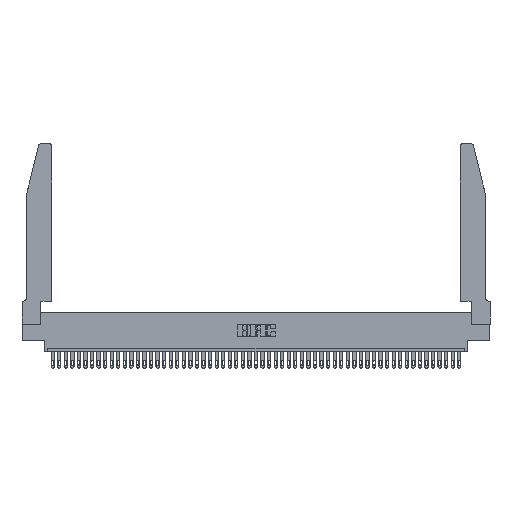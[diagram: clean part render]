
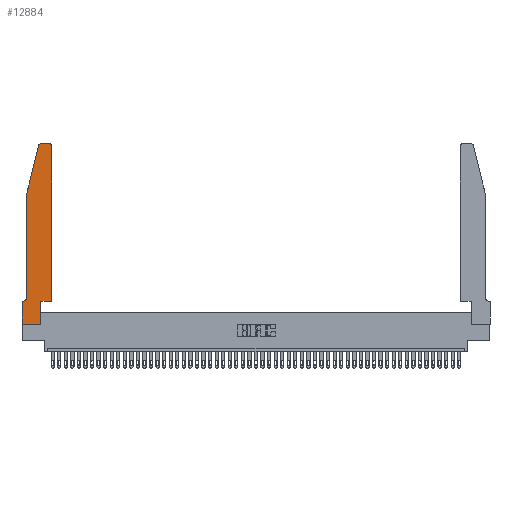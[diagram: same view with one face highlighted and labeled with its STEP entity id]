
A CAD part, top view. The second image highlights one B-rep face of the part: STEP entity #12884.
In plain terms, the highlighted planar face has unit normal (0, 0, 1).
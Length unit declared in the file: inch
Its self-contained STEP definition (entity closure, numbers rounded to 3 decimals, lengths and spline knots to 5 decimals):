
#888 = VERTEX_POINT ( 'NONE', #4504 ) ;
#1213 = DIRECTION ( 'NONE',  ( 0., -1., 0. ) ) ;
#1390 = CIRCLE ( 'NONE', #10165, 0.03 ) ;
#1454 = EDGE_CURVE ( 'NONE', #31015, #30696, #16986, .T. ) ;
#2493 = DIRECTION ( 'NONE',  ( 0., 0., 1. ) ) ;
#2684 = DIRECTION ( 'NONE',  ( 1., 0., 0. ) ) ;
#2699 = ORIENTED_EDGE ( 'NONE', *, *, #43784, .T. ) ;
#3818 = AXIS2_PLACEMENT_3D ( 'NONE', #6189, #2493, #9884 ) ;
#4504 = CARTESIAN_POINT ( 'NONE',  ( 0., 0.35, 0.37 ) ) ;
#4913 = ORIENTED_EDGE ( 'NONE', *, *, #13318, .T. ) ;
#5600 = VECTOR ( 'NONE', #31798, 39.37008 ) ;
#5611 = LINE ( 'NONE', #37325, #37312 ) ;
#5988 = VERTEX_POINT ( 'NONE', #7144 ) ;
#5996 = CARTESIAN_POINT ( 'NONE',  ( 0.0755, 0.42, 0.37 ) ) ;
#6189 = CARTESIAN_POINT ( 'NONE',  ( 0.284, 2.72, 0.37 ) ) ;
#6255 = EDGE_CURVE ( 'NONE', #40191, #6283, #39268, .T. ) ;
#6283 = VERTEX_POINT ( 'NONE', #18095 ) ;
#6309 = DIRECTION ( 'NONE',  ( 1., 0., 0. ) ) ;
#6886 = LINE ( 'NONE', #18804, #15251 ) ;
#7144 = CARTESIAN_POINT ( 'NONE',  ( 0.0055, 0.35, 0.37 ) ) ;
#7612 = CARTESIAN_POINT ( 'NONE',  ( 0.2865, 0., 0.37 ) ) ;
#8094 = EDGE_CURVE ( 'NONE', #49021, #15102, #6886, .T. ) ;
#8491 = CARTESIAN_POINT ( 'NONE',  ( 0.4505, 0.35, 0.37 ) ) ;
#8656 = LINE ( 'NONE', #8491, #48115 ) ;
#8812 = VECTOR ( 'NONE', #42785, 39.37008 ) ;
#9861 = EDGE_CURVE ( 'NONE', #43512, #14122, #1390, .T. ) ;
#9884 = DIRECTION ( 'NONE',  ( 1., 0., 0. ) ) ;
#10165 = AXIS2_PLACEMENT_3D ( 'NONE', #17005, #29199, #6309 ) ;
#10758 = VECTOR ( 'NONE', #1213, 39.37008 ) ;
#11396 = AXIS2_PLACEMENT_3D ( 'NONE', #46126, #45983, #34969 ) ;
#11564 = CARTESIAN_POINT ( 'NONE',  ( 0.0755, 2., 0.37 ) ) ;
#12884 = ADVANCED_FACE ( 'NONE', ( #32865 ), #49000, .T. ) ;
#13318 = EDGE_CURVE ( 'NONE', #888, #31015, #15512, .T. ) ;
#14122 = VERTEX_POINT ( 'NONE', #23144 ) ;
#14564 = CARTESIAN_POINT ( 'NONE',  ( 0.2865, 0.35, 0.37 ) ) ;
#14869 = VECTOR ( 'NONE', #49241, 39.37008 ) ;
#15102 = VERTEX_POINT ( 'NONE', #11564 ) ;
#15251 = VECTOR ( 'NONE', #37318, 39.37008 ) ;
#15512 = LINE ( 'NONE', #32156, #10758 ) ;
#16405 = VECTOR ( 'NONE', #33693, 39.37008 ) ;
#16986 = LINE ( 'NONE', #24149, #5600 ) ;
#17005 = CARTESIAN_POINT ( 'NONE',  ( 0.4205, 2.72, 0.37 ) ) ;
#17025 = EDGE_CURVE ( 'NONE', #6283, #43512, #8656, .T. ) ;
#17609 = DIRECTION ( 'NONE',  ( 0., 0., 1. ) ) ;
#17669 = LINE ( 'NONE', #14564, #16405 ) ;
#18095 = CARTESIAN_POINT ( 'NONE',  ( 0.4505, 0.35, 0.37 ) ) ;
#18153 = CARTESIAN_POINT ( 'NONE',  ( 0.0755, 0.35, 0.37 ) ) ;
#18410 = CARTESIAN_POINT ( 'NONE',  ( 0.2865, 0.35, 0.37 ) ) ;
#18804 = CARTESIAN_POINT ( 'NONE',  ( 0.0755, 2., 0.37 ) ) ;
#19162 = CIRCLE ( 'NONE', #11396, 0.07 ) ;
#19190 = ORIENTED_EDGE ( 'NONE', *, *, #24174, .T. ) ;
#19346 = CARTESIAN_POINT ( 'NONE',  ( 0.25487, 2.72718, 0.37 ) ) ;
#19467 = CARTESIAN_POINT ( 'NONE',  ( 0., 0.35, 0.37 ) ) ;
#20998 = ORIENTED_EDGE ( 'NONE', *, *, #32439, .T. ) ;
#21939 = LINE ( 'NONE', #18153, #40977 ) ;
#21992 = DIRECTION ( 'NONE',  ( -1., 0., 0. ) ) ;
#23144 = CARTESIAN_POINT ( 'NONE',  ( 0.4205, 2.75, 0.37 ) ) ;
#24149 = CARTESIAN_POINT ( 'NONE',  ( 0., 0., 0.37 ) ) ;
#24174 = EDGE_CURVE ( 'NONE', #30195, #49021, #41210, .T. ) ;
#24372 = CARTESIAN_POINT ( 'NONE',  ( 0.4505, 0.35, 0.37 ) ) ;
#26081 = EDGE_CURVE ( 'NONE', #5988, #888, #21939, .T. ) ;
#26747 = ORIENTED_EDGE ( 'NONE', *, *, #8094, .T. ) ;
#26897 = ORIENTED_EDGE ( 'NONE', *, *, #41486, .T. ) ;
#28063 = CARTESIAN_POINT ( 'NONE',  ( 0., 0., 0.37 ) ) ;
#28498 = AXIS2_PLACEMENT_3D ( 'NONE', #19467, #17609, #2684 ) ;
#28583 = DIRECTION ( 'NONE',  ( 0., 1., 0. ) ) ;
#29199 = DIRECTION ( 'NONE',  ( 0., 0., 1. ) ) ;
#29377 = ORIENTED_EDGE ( 'NONE', *, *, #1454, .T. ) ;
#30195 = VERTEX_POINT ( 'NONE', #48517 ) ;
#30696 = VERTEX_POINT ( 'NONE', #7612 ) ;
#31015 = VERTEX_POINT ( 'NONE', #28063 ) ;
#31034 = EDGE_CURVE ( 'NONE', #15102, #44499, #39200, .T. ) ;
#31492 = EDGE_LOOP ( 'NONE', ( #26897, #19190, #26747, #42986, #2699, #42003, #4913, #29377, #20998, #33601, #38681, #46062 ) ) ;
#31798 = DIRECTION ( 'NONE',  ( 1., 0., 0. ) ) ;
#32156 = CARTESIAN_POINT ( 'NONE',  ( 0., 0., 0.37 ) ) ;
#32439 = EDGE_CURVE ( 'NONE', #30696, #40191, #17669, .T. ) ;
#32865 = FACE_OUTER_BOUND ( 'NONE', #31492, .T. ) ;
#33601 = ORIENTED_EDGE ( 'NONE', *, *, #6255, .T. ) ;
#33693 = DIRECTION ( 'NONE',  ( 0., 1., 0. ) ) ;
#34969 = DIRECTION ( 'NONE',  ( -1., 0., 0. ) ) ;
#37312 = VECTOR ( 'NONE', #44972, 39.37008 ) ;
#37318 = DIRECTION ( 'NONE',  ( -0.239, -0.971, 0. ) ) ;
#37325 = CARTESIAN_POINT ( 'NONE',  ( 0.2605, 2.75, 0.37 ) ) ;
#38681 = ORIENTED_EDGE ( 'NONE', *, *, #17025, .T. ) ;
#39200 = LINE ( 'NONE', #44266, #14869 ) ;
#39268 = LINE ( 'NONE', #24372, #8812 ) ;
#40191 = VERTEX_POINT ( 'NONE', #18410 ) ;
#40977 = VECTOR ( 'NONE', #21992, 39.37008 ) ;
#41210 = CIRCLE ( 'NONE', #3818, 0.03 ) ;
#41486 = EDGE_CURVE ( 'NONE', #14122, #30195, #5611, .T. ) ;
#42003 = ORIENTED_EDGE ( 'NONE', *, *, #26081, .T. ) ;
#42785 = DIRECTION ( 'NONE',  ( 1., 0., 0. ) ) ;
#42986 = ORIENTED_EDGE ( 'NONE', *, *, #31034, .T. ) ;
#43512 = VERTEX_POINT ( 'NONE', #44886 ) ;
#43784 = EDGE_CURVE ( 'NONE', #44499, #5988, #19162, .T. ) ;
#44266 = CARTESIAN_POINT ( 'NONE',  ( 0.0755, 2., 0.37 ) ) ;
#44499 = VERTEX_POINT ( 'NONE', #5996 ) ;
#44886 = CARTESIAN_POINT ( 'NONE',  ( 0.4505, 2.72, 0.37 ) ) ;
#44972 = DIRECTION ( 'NONE',  ( -1., 0., 0. ) ) ;
#45983 = DIRECTION ( 'NONE',  ( 0., 0., -1. ) ) ;
#46062 = ORIENTED_EDGE ( 'NONE', *, *, #9861, .T. ) ;
#46126 = CARTESIAN_POINT ( 'NONE',  ( 0.0055, 0.42, 0.37 ) ) ;
#48115 = VECTOR ( 'NONE', #28583, 39.37008 ) ;
#48517 = CARTESIAN_POINT ( 'NONE',  ( 0.284, 2.75, 0.37 ) ) ;
#49000 = PLANE ( 'NONE',  #28498 ) ;
#49021 = VERTEX_POINT ( 'NONE', #19346 ) ;
#49241 = DIRECTION ( 'NONE',  ( 0., -1., 0. ) ) ;
